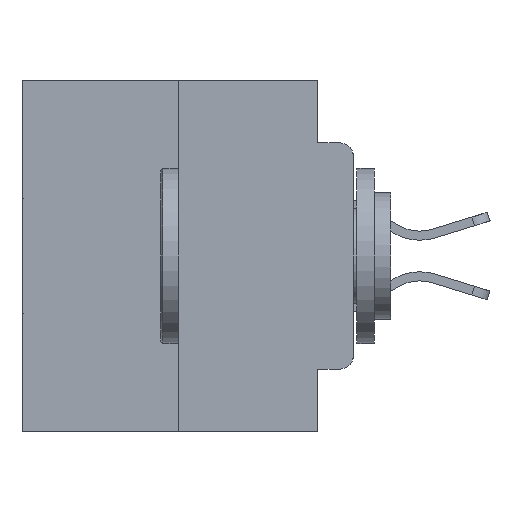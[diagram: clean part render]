
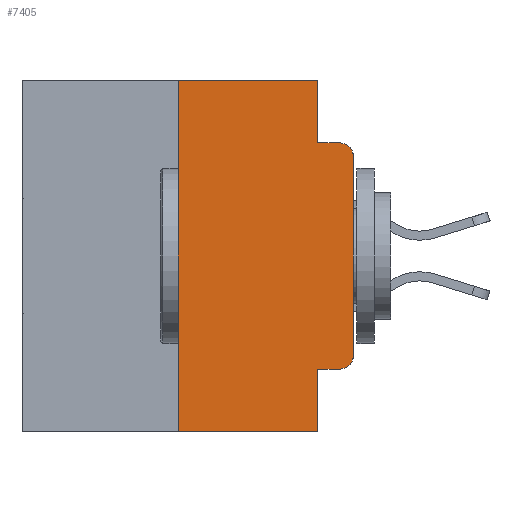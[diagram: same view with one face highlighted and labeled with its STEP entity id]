
A CAD part, left-side view. The second image highlights one B-rep face of the part: STEP entity #7405.
In plain terms, the highlighted planar face has unit normal (-1, 0, 0).
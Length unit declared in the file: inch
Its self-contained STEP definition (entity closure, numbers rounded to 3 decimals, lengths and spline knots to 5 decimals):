
#135 = CARTESIAN_POINT ( 'NONE',  ( 0., 0., -0.3915 ) ) ;
#461 = EDGE_CURVE ( 'NONE', #7030, #19107, #27353, .T. ) ;
#987 = CARTESIAN_POINT ( 'NONE',  ( 0., 0.473, 0. ) ) ;
#1113 = ORIENTED_EDGE ( 'NONE', *, *, #11671, .F. ) ;
#2719 = CARTESIAN_POINT ( 'NONE',  ( 0., 0.051, -0.0885 ) ) ;
#2754 = ORIENTED_EDGE ( 'NONE', *, *, #25116, .T. ) ;
#2909 = VERTEX_POINT ( 'NONE', #25169 ) ;
#3104 = CARTESIAN_POINT ( 'NONE',  ( 0., 0.051, -0.0885 ) ) ;
#3299 = CARTESIAN_POINT ( 'NONE',  ( 0., 0.25, 0. ) ) ;
#3468 = CARTESIAN_POINT ( 'NONE',  ( 0., 0.25, -0.5 ) ) ;
#3589 = EDGE_CURVE ( 'NONE', #2909, #20482, #22591, .T. ) ;
#3730 = VERTEX_POINT ( 'NONE', #3801 ) ;
#3801 = CARTESIAN_POINT ( 'NONE',  ( 0., 0.051, -0.4115 ) ) ;
#3859 = ORIENTED_EDGE ( 'NONE', *, *, #25478, .F. ) ;
#4074 = AXIS2_PLACEMENT_3D ( 'NONE', #14610, #14309, #14014 ) ;
#4413 = VECTOR ( 'NONE', #5855, 39.37008 ) ;
#4636 = ORIENTED_EDGE ( 'NONE', *, *, #6253, .F. ) ;
#5337 = DIRECTION ( 'NONE',  ( -1., 0., 0. ) ) ;
#5779 = LINE ( 'NONE', #16121, #29135 ) ;
#5855 = DIRECTION ( 'NONE',  ( 0., 0., -1. ) ) ;
#6253 = EDGE_CURVE ( 'NONE', #17182, #2909, #13461, .T. ) ;
#6336 = CARTESIAN_POINT ( 'NONE',  ( 0., 0.02, -0.4115 ) ) ;
#6670 = EDGE_CURVE ( 'NONE', #19107, #7267, #14143, .T. ) ;
#7030 = VERTEX_POINT ( 'NONE', #135 ) ;
#7246 = DIRECTION ( 'NONE',  ( 0., 0., 1. ) ) ;
#7267 = VERTEX_POINT ( 'NONE', #25731 ) ;
#7405 = ADVANCED_FACE ( 'NONE', ( #25028 ), #23847, .F. ) ;
#10138 = CARTESIAN_POINT ( 'NONE',  ( 0., 0.473, -0.5 ) ) ;
#10500 = ORIENTED_EDGE ( 'NONE', *, *, #23408, .F. ) ;
#10545 = VERTEX_POINT ( 'NONE', #25650 ) ;
#11102 = EDGE_CURVE ( 'NONE', #16722, #7030, #18021, .T. ) ;
#11671 = EDGE_CURVE ( 'NONE', #20482, #7267, #21830, .T. ) ;
#12023 = CARTESIAN_POINT ( 'NONE',  ( 0., 0., -0.1085 ) ) ;
#12462 = DIRECTION ( 'NONE',  ( 0., -1., 0. ) ) ;
#12568 = VECTOR ( 'NONE', #12462, 39.37008 ) ;
#13461 = LINE ( 'NONE', #987, #18810 ) ;
#13569 = DIRECTION ( 'NONE',  ( 0., 0., -1. ) ) ;
#13738 = DIRECTION ( 'NONE',  ( 0., 0., 1. ) ) ;
#14014 = DIRECTION ( 'NONE',  ( 0., 0., -1. ) ) ;
#14143 = CIRCLE ( 'NONE', #4074, 0.02 ) ;
#14309 = DIRECTION ( 'NONE',  ( -1., 0., 0. ) ) ;
#14610 = CARTESIAN_POINT ( 'NONE',  ( 0., 0.02, -0.1085 ) ) ;
#15166 = VECTOR ( 'NONE', #20872, 39.37008 ) ;
#16121 = CARTESIAN_POINT ( 'NONE',  ( 0., 0.051, -0.4115 ) ) ;
#16181 = CARTESIAN_POINT ( 'NONE',  ( 0., 0.051, 0. ) ) ;
#16325 = ORIENTED_EDGE ( 'NONE', *, *, #11102, .T. ) ;
#16722 = VERTEX_POINT ( 'NONE', #6336 ) ;
#17182 = VERTEX_POINT ( 'NONE', #3299 ) ;
#18021 = CIRCLE ( 'NONE', #28103, 0.02 ) ;
#18045 = ORIENTED_EDGE ( 'NONE', *, *, #461, .T. ) ;
#18810 = VECTOR ( 'NONE', #24632, 39.37008 ) ;
#19064 = CARTESIAN_POINT ( 'NONE',  ( 0., 0.02, -0.3915 ) ) ;
#19107 = VERTEX_POINT ( 'NONE', #12023 ) ;
#19651 = VECTOR ( 'NONE', #13738, 39.37008 ) ;
#20482 = VERTEX_POINT ( 'NONE', #3104 ) ;
#20872 = DIRECTION ( 'NONE',  ( 0., -1., 0. ) ) ;
#21221 = VERTEX_POINT ( 'NONE', #3468 ) ;
#21244 = CARTESIAN_POINT ( 'NONE',  ( 0., 0., 0. ) ) ;
#21287 = DIRECTION ( 'NONE',  ( 0., 0., -1. ) ) ;
#21363 = VECTOR ( 'NONE', #7246, 39.37008 ) ;
#21778 = LINE ( 'NONE', #27072, #29114 ) ;
#21830 = LINE ( 'NONE', #2719, #15166 ) ;
#22501 = ORIENTED_EDGE ( 'NONE', *, *, #22857, .T. ) ;
#22591 = LINE ( 'NONE', #16181, #4413 ) ;
#22857 = EDGE_CURVE ( 'NONE', #3730, #16722, #5779, .T. ) ;
#23171 = LINE ( 'NONE', #10138, #12568 ) ;
#23408 = EDGE_CURVE ( 'NONE', #3730, #10545, #21778, .T. ) ;
#23615 = DIRECTION ( 'NONE',  ( 0., 0., -1. ) ) ;
#23654 = DIRECTION ( 'NONE',  ( 1., 0., 0. ) ) ;
#23688 = CARTESIAN_POINT ( 'NONE',  ( 0., 0.473, 0. ) ) ;
#23847 = PLANE ( 'NONE',  #25800 ) ;
#24632 = DIRECTION ( 'NONE',  ( 0., -1., 0. ) ) ;
#25028 = FACE_OUTER_BOUND ( 'NONE', #25610, .T. ) ;
#25095 = ORIENTED_EDGE ( 'NONE', *, *, #6670, .T. ) ;
#25116 = EDGE_CURVE ( 'NONE', #21221, #10545, #23171, .T. ) ;
#25140 = DIRECTION ( 'NONE',  ( 0., -1., 0. ) ) ;
#25169 = CARTESIAN_POINT ( 'NONE',  ( 0., 0.051, 0. ) ) ;
#25478 = EDGE_CURVE ( 'NONE', #21221, #17182, #25622, .T. ) ;
#25610 = EDGE_LOOP ( 'NONE', ( #18045, #25095, #1113, #26742, #4636, #3859, #2754, #10500, #22501, #16325 ) ) ;
#25622 = LINE ( 'NONE', #27242, #19651 ) ;
#25650 = CARTESIAN_POINT ( 'NONE',  ( 0., 0.051, -0.5 ) ) ;
#25731 = CARTESIAN_POINT ( 'NONE',  ( 0., 0.02, -0.0885 ) ) ;
#25800 = AXIS2_PLACEMENT_3D ( 'NONE', #23688, #23654, #23615 ) ;
#26742 = ORIENTED_EDGE ( 'NONE', *, *, #3589, .F. ) ;
#27072 = CARTESIAN_POINT ( 'NONE',  ( 0., 0.051, 0. ) ) ;
#27242 = CARTESIAN_POINT ( 'NONE',  ( 0., 0.25, 0. ) ) ;
#27353 = LINE ( 'NONE', #21244, #21363 ) ;
#28103 = AXIS2_PLACEMENT_3D ( 'NONE', #19064, #5337, #21287 ) ;
#29114 = VECTOR ( 'NONE', #13569, 39.37008 ) ;
#29135 = VECTOR ( 'NONE', #25140, 39.37008 ) ;
